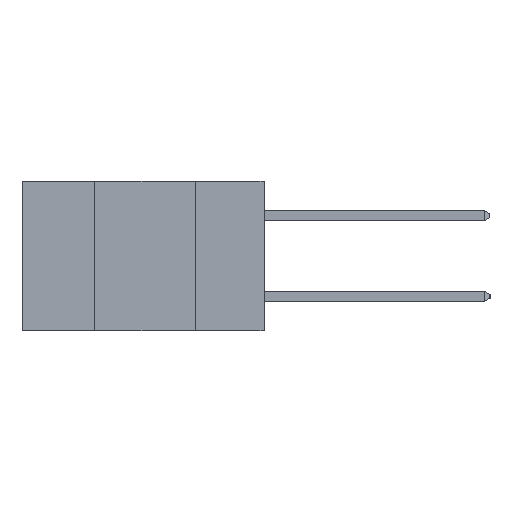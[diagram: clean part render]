
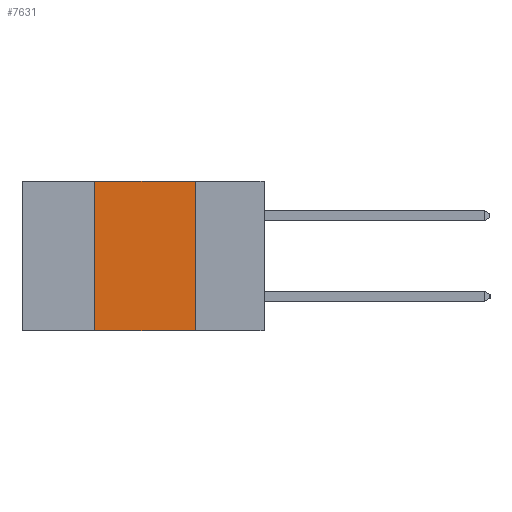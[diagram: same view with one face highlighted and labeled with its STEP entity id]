
A CAD part, left-side view. The second image highlights one B-rep face of the part: STEP entity #7631.
In plain terms, the highlighted planar face has unit normal (-1, 0, 0).
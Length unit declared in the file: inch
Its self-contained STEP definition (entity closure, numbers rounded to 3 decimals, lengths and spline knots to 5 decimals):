
#726 = VECTOR ( 'NONE', #16012, 39.37008 ) ;
#1207 = CARTESIAN_POINT ( 'NONE',  ( 0., 0.17, -0.37 ) ) ;
#1261 = EDGE_LOOP ( 'NONE', ( #18543, #25241, #17031, #16107 ) ) ;
#2861 = VERTEX_POINT ( 'NONE', #19224 ) ;
#3147 = DIRECTION ( 'NONE',  ( 0., 0., -1. ) ) ;
#3848 = CARTESIAN_POINT ( 'NONE',  ( 0., 0.42, 0. ) ) ;
#3893 = CARTESIAN_POINT ( 'NONE',  ( 0., 0.6, -0.37 ) ) ;
#4680 = VERTEX_POINT ( 'NONE', #23268 ) ;
#5208 = EDGE_CURVE ( 'NONE', #22257, #4680, #11082, .T. ) ;
#5603 = VECTOR ( 'NONE', #15669, 39.37008 ) ;
#6731 = VECTOR ( 'NONE', #19255, 39.37008 ) ;
#7356 = CARTESIAN_POINT ( 'NONE',  ( 0., 0.42, -0.37 ) ) ;
#7631 = ADVANCED_FACE ( 'NONE', ( #12162 ), #13669, .F. ) ;
#10607 = VERTEX_POINT ( 'NONE', #7356 ) ;
#10626 = EDGE_CURVE ( 'NONE', #10607, #22257, #11996, .T. ) ;
#10825 = LINE ( 'NONE', #1207, #20696 ) ;
#11082 = LINE ( 'NONE', #16852, #726 ) ;
#11996 = LINE ( 'NONE', #21133, #6731 ) ;
#12162 = FACE_OUTER_BOUND ( 'NONE', #1261, .T. ) ;
#13615 = DIRECTION ( 'NONE',  ( 0., 0., -1. ) ) ;
#13635 = DIRECTION ( 'NONE',  ( 1., 0., 0. ) ) ;
#13642 = CARTESIAN_POINT ( 'NONE',  ( 0., 0.6, 0. ) ) ;
#13669 = PLANE ( 'NONE',  #15151 ) ;
#15151 = AXIS2_PLACEMENT_3D ( 'NONE', #13642, #13635, #13615 ) ;
#15669 = DIRECTION ( 'NONE',  ( 0., -1., 0. ) ) ;
#16012 = DIRECTION ( 'NONE',  ( 0., -1., 0. ) ) ;
#16107 = ORIENTED_EDGE ( 'NONE', *, *, #18620, .T. ) ;
#16852 = CARTESIAN_POINT ( 'NONE',  ( 0., 0.6, 0. ) ) ;
#17031 = ORIENTED_EDGE ( 'NONE', *, *, #10626, .F. ) ;
#18543 = ORIENTED_EDGE ( 'NONE', *, *, #19076, .F. ) ;
#18620 = EDGE_CURVE ( 'NONE', #10607, #2861, #21318, .T. ) ;
#19076 = EDGE_CURVE ( 'NONE', #4680, #2861, #10825, .T. ) ;
#19224 = CARTESIAN_POINT ( 'NONE',  ( 0., 0.17, -0.37 ) ) ;
#19255 = DIRECTION ( 'NONE',  ( 0., 0., 1. ) ) ;
#20696 = VECTOR ( 'NONE', #3147, 39.37008 ) ;
#21133 = CARTESIAN_POINT ( 'NONE',  ( 0., 0.42, -0.37 ) ) ;
#21318 = LINE ( 'NONE', #3893, #5603 ) ;
#22257 = VERTEX_POINT ( 'NONE', #3848 ) ;
#23268 = CARTESIAN_POINT ( 'NONE',  ( 0., 0.17, 0. ) ) ;
#25241 = ORIENTED_EDGE ( 'NONE', *, *, #5208, .F. ) ;
